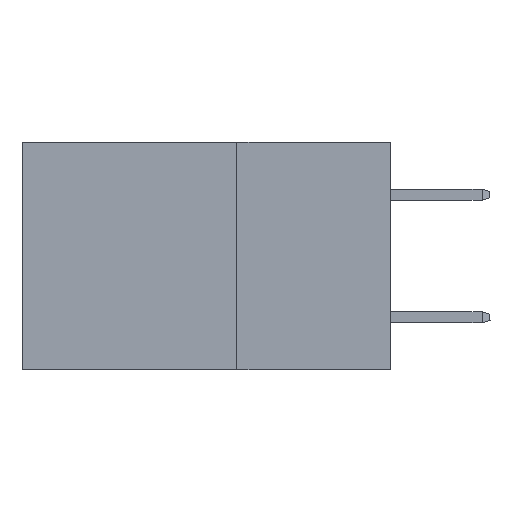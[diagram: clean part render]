
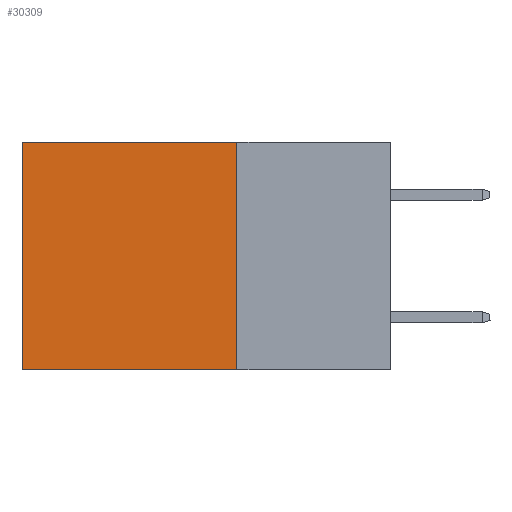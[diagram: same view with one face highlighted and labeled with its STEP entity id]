
A CAD part, left-side view. The second image highlights one B-rep face of the part: STEP entity #30309.
In plain terms, the highlighted planar face has unit normal (-1, 0, 0).
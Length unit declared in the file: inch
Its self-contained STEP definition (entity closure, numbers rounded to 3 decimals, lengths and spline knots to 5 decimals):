
#1086 = ORIENTED_EDGE ( 'NONE', *, *, #16622, .T. ) ;
#1356 = VECTOR ( 'NONE', #13443, 39.37008 ) ;
#1454 = LINE ( 'NONE', #17103, #25777 ) ;
#1527 = AXIS2_PLACEMENT_3D ( 'NONE', #8423, #14193, #30393 ) ;
#1549 = VERTEX_POINT ( 'NONE', #26041 ) ;
#2917 = CARTESIAN_POINT ( 'NONE',  ( 0.2875, 0.6, 0. ) ) ;
#3318 = FACE_OUTER_BOUND ( 'NONE', #16723, .T. ) ;
#4573 = VECTOR ( 'NONE', #23063, 39.37008 ) ;
#7067 = EDGE_CURVE ( 'NONE', #14427, #20979, #9173, .T. ) ;
#8423 = CARTESIAN_POINT ( 'NONE',  ( 0.2875, 0.25, 0. ) ) ;
#9173 = LINE ( 'NONE', #11469, #34066 ) ;
#11469 = CARTESIAN_POINT ( 'NONE',  ( 0.2875, 0.25, -0.37 ) ) ;
#12146 = CARTESIAN_POINT ( 'NONE',  ( 0.2875, 0.25, 0. ) ) ;
#13443 = DIRECTION ( 'NONE',  ( 0., 0., -1. ) ) ;
#14193 = DIRECTION ( 'NONE',  ( 1., 0., 0. ) ) ;
#14427 = VERTEX_POINT ( 'NONE', #32553 ) ;
#14442 = LINE ( 'NONE', #12146, #4573 ) ;
#15250 = CARTESIAN_POINT ( 'NONE',  ( 0.2875, 0.6, -0.37 ) ) ;
#15334 = CARTESIAN_POINT ( 'NONE',  ( 0.2875, 0.6, 0. ) ) ;
#15579 = LINE ( 'NONE', #2917, #1356 ) ;
#16622 = EDGE_CURVE ( 'NONE', #25727, #20979, #15579, .T. ) ;
#16723 = EDGE_LOOP ( 'NONE', ( #1086, #30382, #31677, #31693 ) ) ;
#17103 = CARTESIAN_POINT ( 'NONE',  ( 0.2875, 0.25, 0. ) ) ;
#20979 = VERTEX_POINT ( 'NONE', #15250 ) ;
#23063 = DIRECTION ( 'NONE',  ( 0., 1., 0. ) ) ;
#25727 = VERTEX_POINT ( 'NONE', #15334 ) ;
#25777 = VECTOR ( 'NONE', #33492, 39.37008 ) ;
#26041 = CARTESIAN_POINT ( 'NONE',  ( 0.2875, 0.25, 0. ) ) ;
#27577 = PLANE ( 'NONE',  #1527 ) ;
#28415 = EDGE_CURVE ( 'NONE', #1549, #25727, #14442, .T. ) ;
#30309 = ADVANCED_FACE ( 'NONE', ( #3318 ), #27577, .F. ) ;
#30382 = ORIENTED_EDGE ( 'NONE', *, *, #7067, .F. ) ;
#30393 = DIRECTION ( 'NONE',  ( 0., 0., -1. ) ) ;
#31677 = ORIENTED_EDGE ( 'NONE', *, *, #34010, .F. ) ;
#31693 = ORIENTED_EDGE ( 'NONE', *, *, #28415, .T. ) ;
#32553 = CARTESIAN_POINT ( 'NONE',  ( 0.2875, 0.25, -0.37 ) ) ;
#32951 = DIRECTION ( 'NONE',  ( 0., 1., 0. ) ) ;
#33492 = DIRECTION ( 'NONE',  ( 0., 0., -1. ) ) ;
#34010 = EDGE_CURVE ( 'NONE', #1549, #14427, #1454, .T. ) ;
#34066 = VECTOR ( 'NONE', #32951, 39.37008 ) ;
